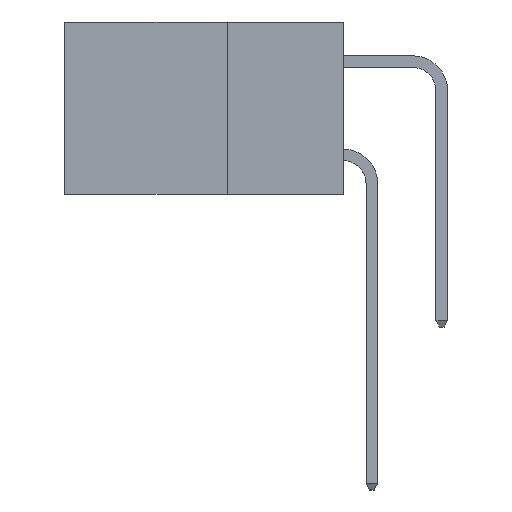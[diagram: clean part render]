
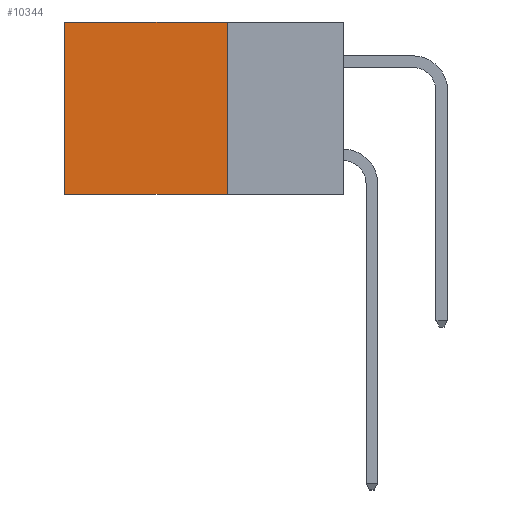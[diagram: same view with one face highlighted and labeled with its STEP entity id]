
A CAD part, left-side view. The second image highlights one B-rep face of the part: STEP entity #10344.
In plain terms, the highlighted planar face has unit normal (-1, 0, 0).
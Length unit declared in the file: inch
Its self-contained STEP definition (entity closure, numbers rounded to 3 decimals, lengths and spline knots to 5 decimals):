
#515 = CARTESIAN_POINT ( 'NONE',  ( 0.2615, 0.6, -0.37 ) ) ;
#1065 = VECTOR ( 'NONE', #16553, 39.37008 ) ;
#1490 = EDGE_CURVE ( 'NONE', #11671, #20069, #18112, .T. ) ;
#1636 = CARTESIAN_POINT ( 'NONE',  ( 0.2615, 0.6, 0. ) ) ;
#1717 = CARTESIAN_POINT ( 'NONE',  ( 0.2615, 0.25, -0.37 ) ) ;
#2390 = AXIS2_PLACEMENT_3D ( 'NONE', #5274, #16392, #6889 ) ;
#2548 = DIRECTION ( 'NONE',  ( 0., 1., 0. ) ) ;
#3693 = ORIENTED_EDGE ( 'NONE', *, *, #14558, .F. ) ;
#3783 = LINE ( 'NONE', #1717, #19639 ) ;
#5274 = CARTESIAN_POINT ( 'NONE',  ( 0.2615, 0.25, -0.37 ) ) ;
#5431 = LINE ( 'NONE', #7069, #1065 ) ;
#6643 = DIRECTION ( 'NONE',  ( 0., 0., -1. ) ) ;
#6889 = DIRECTION ( 'NONE',  ( 0., 0., -1. ) ) ;
#7069 = CARTESIAN_POINT ( 'NONE',  ( 0.2615, 0.6, -0.37 ) ) ;
#7207 = ORIENTED_EDGE ( 'NONE', *, *, #13439, .F. ) ;
#8154 = CARTESIAN_POINT ( 'NONE',  ( 0.2615, 0.25, 0. ) ) ;
#8782 = LINE ( 'NONE', #9500, #19836 ) ;
#9500 = CARTESIAN_POINT ( 'NONE',  ( 0.2615, 0.25, -0.37 ) ) ;
#10344 = ADVANCED_FACE ( 'NONE', ( #19290 ), #13241, .F. ) ;
#11072 = VERTEX_POINT ( 'NONE', #13347 ) ;
#11671 = VERTEX_POINT ( 'NONE', #17980 ) ;
#13241 = PLANE ( 'NONE',  #2390 ) ;
#13347 = CARTESIAN_POINT ( 'NONE',  ( 0.2615, 0.25, -0.37 ) ) ;
#13439 = EDGE_CURVE ( 'NONE', #11671, #11072, #3783, .T. ) ;
#14558 = EDGE_CURVE ( 'NONE', #11072, #15808, #8782, .T. ) ;
#14597 = ORIENTED_EDGE ( 'NONE', *, *, #19651, .T. ) ;
#14599 = EDGE_LOOP ( 'NONE', ( #14597, #3693, #7207, #15631 ) ) ;
#15631 = ORIENTED_EDGE ( 'NONE', *, *, #1490, .T. ) ;
#15808 = VERTEX_POINT ( 'NONE', #515 ) ;
#15851 = DIRECTION ( 'NONE',  ( 0., 1., 0. ) ) ;
#16392 = DIRECTION ( 'NONE',  ( 1., 0., 0. ) ) ;
#16553 = DIRECTION ( 'NONE',  ( 0., 0., -1. ) ) ;
#17647 = VECTOR ( 'NONE', #2548, 39.37008 ) ;
#17980 = CARTESIAN_POINT ( 'NONE',  ( 0.2615, 0.25, 0. ) ) ;
#18112 = LINE ( 'NONE', #8154, #17647 ) ;
#19290 = FACE_OUTER_BOUND ( 'NONE', #14599, .T. ) ;
#19639 = VECTOR ( 'NONE', #6643, 39.37008 ) ;
#19651 = EDGE_CURVE ( 'NONE', #20069, #15808, #5431, .T. ) ;
#19836 = VECTOR ( 'NONE', #15851, 39.37008 ) ;
#20069 = VERTEX_POINT ( 'NONE', #1636 ) ;
